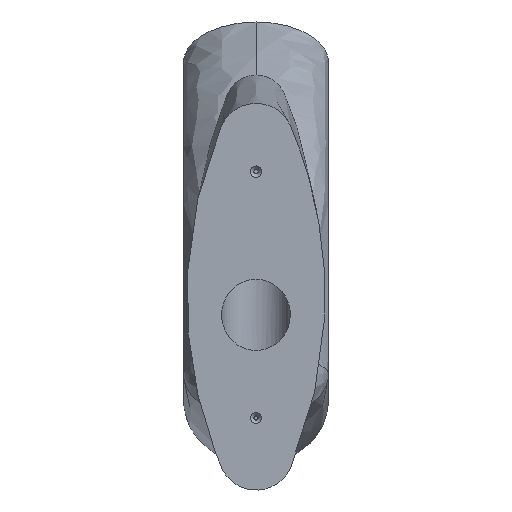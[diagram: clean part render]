
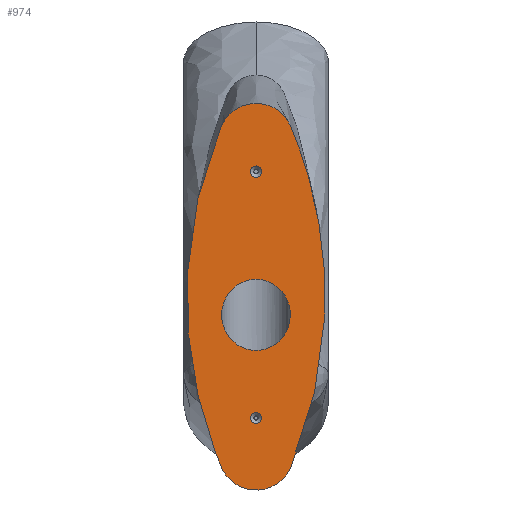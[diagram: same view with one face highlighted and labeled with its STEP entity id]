
A CAD part, front view. The second image highlights one B-rep face of the part: STEP entity #974.
In plain terms, the highlighted planar face has unit normal (0, -1, 0).
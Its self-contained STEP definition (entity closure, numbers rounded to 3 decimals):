
#17=ELLIPSE('',#1040,8.655,8.36);
#20=FACE_BOUND('',#266,.T.);
#21=FACE_BOUND('',#267,.T.);
#22=FACE_BOUND('',#268,.T.);
#113=B_SPLINE_CURVE_WITH_KNOTS('',3,(#3445,#3446,#3447,#3448,#3449,#3450,
#3451,#3452,#3453,#3454,#3455,#3456,#3457,#3458,#3459,#3460,#3461,#3462,
#3463,#3464,#3465,#3466,#3467,#3468,#3469,#3470,#3471,#3472,#3473,#3474,
#3475,#3476,#3477,#3478,#3479,#3480,#3481,#3482,#3483,#3484,#3485,#3486,
#3487,#3488,#3489,#3490,#3491,#3492,#3493,#3494,#3495,#3496),
 .UNSPECIFIED.,.T.,.F.,(4,3,3,3,3,3,3,3,3,3,3,3,3,3,3,3,3,4),(-22.154,
-21.595,-21.036,-20.477,-19.919,
-18.814,-17.709,-15.499,-13.289,
-11.079,-10.519,-9.959,-9.4,
-8.84,-6.63,-4.42,-2.21,
0.),.UNSPECIFIED.);
#143=PLANE('',#1042);
#204=FACE_OUTER_BOUND('',#265,.T.);
#265=EDGE_LOOP('',(#866));
#266=EDGE_LOOP('',(#867));
#267=EDGE_LOOP('',(#868));
#268=EDGE_LOOP('',(#869));
#357=CIRCLE('',#991,1.4);
#360=CIRCLE('',#997,1.4);
#388=VERTEX_POINT('',#1221);
#391=VERTEX_POINT('',#1232);
#468=VERTEX_POINT('',#3443);
#479=VERTEX_POINT('',#4306);
#483=EDGE_CURVE('',#388,#388,#357,.T.);
#488=EDGE_CURVE('',#391,#391,#360,.T.);
#598=EDGE_CURVE('',#468,#468,#113,.T.);
#620=EDGE_CURVE('',#479,#479,#17,.T.);
#866=ORIENTED_EDGE('',*,*,#598,.T.);
#867=ORIENTED_EDGE('',*,*,#488,.T.);
#868=ORIENTED_EDGE('',*,*,#483,.T.);
#869=ORIENTED_EDGE('',*,*,#620,.T.);
#974=ADVANCED_FACE('',(#204,#20,#21,#22),#143,.T.);
#991=AXIS2_PLACEMENT_3D('',#1222,#1060,#1061);
#997=AXIS2_PLACEMENT_3D('',#1233,#1074,#1075);
#1040=AXIS2_PLACEMENT_3D('',#4308,#1195,#1196);
#1042=AXIS2_PLACEMENT_3D('',#4310,#1199,#1200);
#1060=DIRECTION('center_axis',(0.,1.,0.));
#1061=DIRECTION('ref_axis',(1.,0.,0.));
#1074=DIRECTION('center_axis',(0.,1.,0.));
#1075=DIRECTION('ref_axis',(1.,0.,0.));
#1195=DIRECTION('center_axis',(0.,1.,0.));
#1196=DIRECTION('ref_axis',(0.,0.,-1.));
#1199=DIRECTION('center_axis',(0.,-1.,0.));
#1200=DIRECTION('ref_axis',(0.,0.,-1.));
#1221=CARTESIAN_POINT('',(-1.4,-195.,-79.44));
#1222=CARTESIAN_POINT('Origin',(0.,-195.,-79.44));
#1232=CARTESIAN_POINT('',(-1.4,-195.,-19.44));
#1233=CARTESIAN_POINT('Origin',(0.,-195.,-19.44));
#3443=CARTESIAN_POINT('',(8.453,-195.,-8.411));
#3445=CARTESIAN_POINT('Ctrl Pts',(8.453,-195.,-8.411));
#3446=CARTESIAN_POINT('Ctrl Pts',(7.795,-195.,-6.855));
#3447=CARTESIAN_POINT('Ctrl Pts',(6.652,-195.,-5.413));
#3448=CARTESIAN_POINT('Ctrl Pts',(5.162,-195.,-4.402));
#3449=CARTESIAN_POINT('Ctrl Pts',(3.673,-195.,-3.392));
#3450=CARTESIAN_POINT('Ctrl Pts',(1.835,-195.,-2.812));
#3451=CARTESIAN_POINT('Ctrl Pts',(-0.001,-195.,-2.812));
#3452=CARTESIAN_POINT('Ctrl Pts',(-1.837,-195.,-2.812));
#3453=CARTESIAN_POINT('Ctrl Pts',(-3.673,-195.,-3.392));
#3454=CARTESIAN_POINT('Ctrl Pts',(-5.162,-195.,-4.403));
#3455=CARTESIAN_POINT('Ctrl Pts',(-6.652,-195.,-5.414));
#3456=CARTESIAN_POINT('Ctrl Pts',(-7.796,-195.,-6.856));
#3457=CARTESIAN_POINT('Ctrl Pts',(-8.453,-195.,-8.412));
#3458=CARTESIAN_POINT('Ctrl Pts',(-9.753,-195.,-11.487));
#3459=CARTESIAN_POINT('Ctrl Pts',(-10.939,-195.,-14.699));
#3460=CARTESIAN_POINT('Ctrl Pts',(-11.979,-195.,-18.019));
#3461=CARTESIAN_POINT('Ctrl Pts',(-13.019,-195.,-21.338));
#3462=CARTESIAN_POINT('Ctrl Pts',(-13.913,-195.,-24.765));
#3463=CARTESIAN_POINT('Ctrl Pts',(-14.636,-195.,-28.268));
#3464=CARTESIAN_POINT('Ctrl Pts',(-16.083,-195.,-35.273));
#3465=CARTESIAN_POINT('Ctrl Pts',(-16.848,-195.,-42.582));
#3466=CARTESIAN_POINT('Ctrl Pts',(-16.85,-195.,-49.893));
#3467=CARTESIAN_POINT('Ctrl Pts',(-16.852,-195.,-57.204));
#3468=CARTESIAN_POINT('Ctrl Pts',(-16.092,-195.,-64.517));
#3469=CARTESIAN_POINT('Ctrl Pts',(-14.644,-195.,-71.525));
#3470=CARTESIAN_POINT('Ctrl Pts',(-13.197,-195.,-78.534));
#3471=CARTESIAN_POINT('Ctrl Pts',(-11.064,-195.,-85.239));
#3472=CARTESIAN_POINT('Ctrl Pts',(-8.465,-195.,-91.396));
#3473=CARTESIAN_POINT('Ctrl Pts',(-7.807,-195.,-92.955));
#3474=CARTESIAN_POINT('Ctrl Pts',(-6.661,-195.,-94.399));
#3475=CARTESIAN_POINT('Ctrl Pts',(-5.169,-195.,-95.411));
#3476=CARTESIAN_POINT('Ctrl Pts',(-3.677,-195.,-96.423));
#3477=CARTESIAN_POINT('Ctrl Pts',(-1.838,-195.,-97.002));
#3478=CARTESIAN_POINT('Ctrl Pts',(0.,-195.,-97.002));
#3479=CARTESIAN_POINT('Ctrl Pts',(1.838,-195.,-97.002));
#3480=CARTESIAN_POINT('Ctrl Pts',(3.676,-195.,-96.423));
#3481=CARTESIAN_POINT('Ctrl Pts',(5.169,-195.,-95.411));
#3482=CARTESIAN_POINT('Ctrl Pts',(6.661,-195.,-94.399));
#3483=CARTESIAN_POINT('Ctrl Pts',(7.807,-195.,-92.955));
#3484=CARTESIAN_POINT('Ctrl Pts',(8.465,-195.,-91.395));
#3485=CARTESIAN_POINT('Ctrl Pts',(11.064,-195.,-85.239));
#3486=CARTESIAN_POINT('Ctrl Pts',(13.196,-195.,-78.533));
#3487=CARTESIAN_POINT('Ctrl Pts',(14.644,-195.,-71.525));
#3488=CARTESIAN_POINT('Ctrl Pts',(16.091,-195.,-64.516));
#3489=CARTESIAN_POINT('Ctrl Pts',(16.853,-195.,-57.205));
#3490=CARTESIAN_POINT('Ctrl Pts',(16.851,-195.,-49.894));
#3491=CARTESIAN_POINT('Ctrl Pts',(16.85,-195.,-42.583));
#3492=CARTESIAN_POINT('Ctrl Pts',(16.084,-195.,-35.273));
#3493=CARTESIAN_POINT('Ctrl Pts',(14.636,-195.,-28.268));
#3494=CARTESIAN_POINT('Ctrl Pts',(13.189,-195.,-21.263));
#3495=CARTESIAN_POINT('Ctrl Pts',(11.058,-195.,-14.563));
#3496=CARTESIAN_POINT('Ctrl Pts',(8.453,-195.,-8.411));
#4306=CARTESIAN_POINT('',(8.36,-195.,-54.318));
#4308=CARTESIAN_POINT('Origin',(0.,-195.,-54.318));
#4310=CARTESIAN_POINT('Origin',(-0.135,-195.,-55.596));
